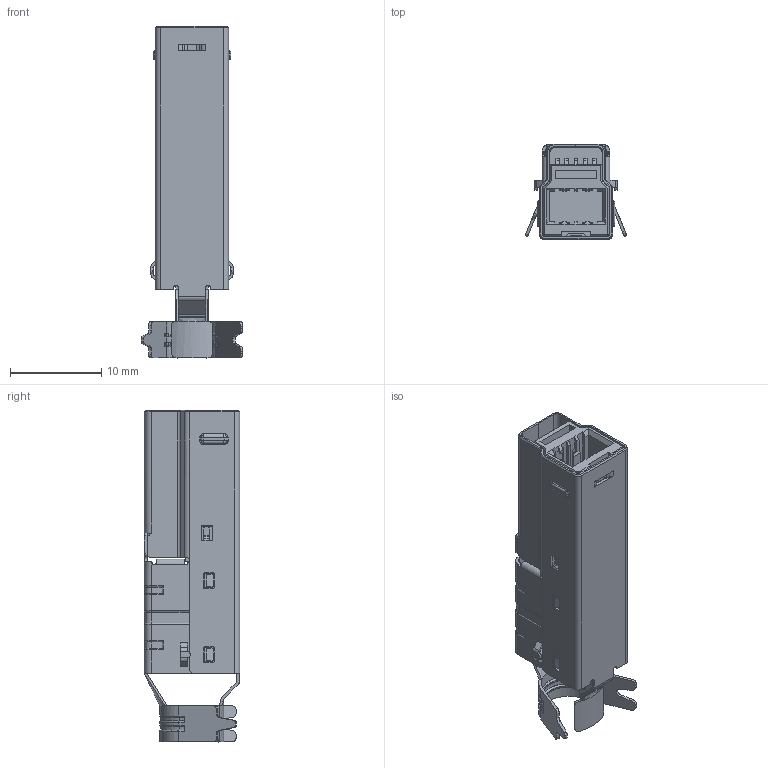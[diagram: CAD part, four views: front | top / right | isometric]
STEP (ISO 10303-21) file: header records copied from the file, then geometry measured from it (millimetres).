
FILE_DESCRIPTION (( 'STEP AP214' ), '1' );
FILE_NAME ('691F209-190-712.STEP', '2021-03-29T19:14:41', ( '' ), ( '' ), 'SwSTEP 2.0', 'SolidWorks 2020', '' );
FILE_SCHEMA (( 'AUTOMOTIVE_DESIGN' ));
Length unit declared in the file: millimetre
Products named in the file (5): Shell 1 691F209-X90-7XX; Shell 2 691F209-X90-7XX; Contacts 691F209-X90-7XX; 691F209-190-712; Insulator 691F209-X90-7XX_Blue
Assembly tree (4 placements, depth 2):
  691F209-190-712
    Insulator 691F209-X90-7XX_Blue
    Shell 2 691F209-X90-7XX
    Shell 1 691F209-X90-7XX
    Contacts 691F209-X90-7XX
Bounding box: 11.11 x 10.44 x 36.3 mm (x, y, z)
Volume: 931.4 mm3; surface area: 3749.7 mm2
Topology: 12 solids, 12 shells, 1476 faces, 4038 edges, 2536 vertices
Faces by surface type: plane 812, cylinder 525, bspline 118, cone 21
Entity records: 49374 total; most frequent: CARTESIAN_POINT 13354, ORIENTED_EDGE 7980, DIRECTION 6806, EDGE_CURVE 3990, VERTEX_POINT 2536, VECTOR 2480, LINE 2480, AXIS2_PLACEMENT_3D 2163
